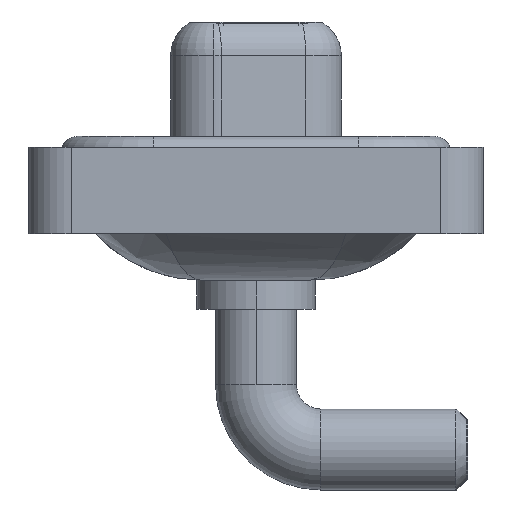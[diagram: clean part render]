
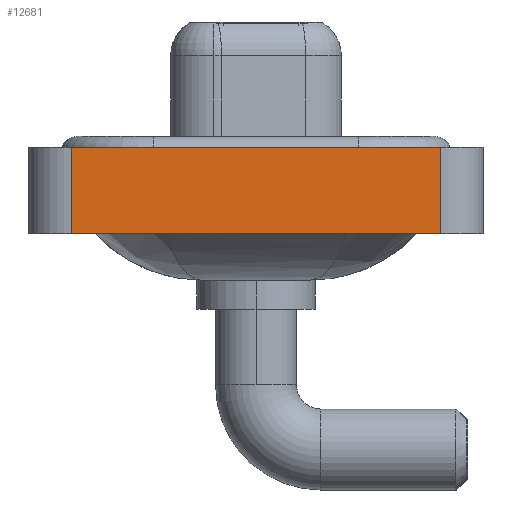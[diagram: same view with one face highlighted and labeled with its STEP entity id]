
A CAD part, left-side view. The second image highlights one B-rep face of the part: STEP entity #12681.
In plain terms, the highlighted planar face has unit normal (-1, 0, 0).
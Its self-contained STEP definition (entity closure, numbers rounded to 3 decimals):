
#26 = ORIENTED_EDGE ( 'NONE', *, *, #15124, .T. ) ;
#262 = VECTOR ( 'NONE', #4863, 1000. ) ;
#936 = PLANE ( 'NONE',  #14161 ) ;
#1154 = ORIENTED_EDGE ( 'NONE', *, *, #9562, .F. ) ;
#1567 = LINE ( 'NONE', #10832, #7258 ) ;
#1940 = VERTEX_POINT ( 'NONE', #12372 ) ;
#2435 = CARTESIAN_POINT ( 'NONE',  ( -7.25, 8.55, -3.6 ) ) ;
#2725 = EDGE_CURVE ( 'NONE', #8722, #10968, #13493, .T. ) ;
#4683 = FACE_OUTER_BOUND ( 'NONE', #9841, .T. ) ;
#4853 = DIRECTION ( 'NONE',  ( -1., 0., 0. ) ) ;
#4863 = DIRECTION ( 'NONE',  ( 0., 0., 1. ) ) ;
#6028 = CARTESIAN_POINT ( 'NONE',  ( -7.25, -8.55, -3.6 ) ) ;
#6979 = CARTESIAN_POINT ( 'NONE',  ( -7.25, 8.55, -3.6 ) ) ;
#7027 = CARTESIAN_POINT ( 'NONE',  ( -7.25, -8.55, -3.6 ) ) ;
#7258 = VECTOR ( 'NONE', #12189, 1000. ) ;
#7540 = DIRECTION ( 'NONE',  ( 0., 0., 1. ) ) ;
#8027 = EDGE_CURVE ( 'NONE', #9073, #1940, #16007, .T. ) ;
#8722 = VERTEX_POINT ( 'NONE', #10783 ) ;
#9073 = VERTEX_POINT ( 'NONE', #2435 ) ;
#9562 = EDGE_CURVE ( 'NONE', #1940, #10968, #16248, .T. ) ;
#9783 = DIRECTION ( 'NONE',  ( 0., -1., 0. ) ) ;
#9841 = EDGE_LOOP ( 'NONE', ( #10234, #1154, #15291, #26 ) ) ;
#10117 = VECTOR ( 'NONE', #7540, 1000. ) ;
#10234 = ORIENTED_EDGE ( 'NONE', *, *, #2725, .T. ) ;
#10783 = CARTESIAN_POINT ( 'NONE',  ( -7.25, -8.55, -3.6 ) ) ;
#10832 = CARTESIAN_POINT ( 'NONE',  ( -7.25, -8.55, -3.6 ) ) ;
#10968 = VERTEX_POINT ( 'NONE', #13185 ) ;
#10972 = CARTESIAN_POINT ( 'NONE',  ( -7.25, -8.55, 0.4 ) ) ;
#12189 = DIRECTION ( 'NONE',  ( 0., -1., 0. ) ) ;
#12372 = CARTESIAN_POINT ( 'NONE',  ( -7.25, 8.55, 0.4 ) ) ;
#12681 = ADVANCED_FACE ( 'NONE', ( #4683 ), #936, .T. ) ;
#13185 = CARTESIAN_POINT ( 'NONE',  ( -7.25, -8.55, 0.4 ) ) ;
#13493 = LINE ( 'NONE', #7027, #10117 ) ;
#14161 = AXIS2_PLACEMENT_3D ( 'NONE', #6028, #4853, #15051 ) ;
#15029 = VECTOR ( 'NONE', #9783, 1000. ) ;
#15051 = DIRECTION ( 'NONE',  ( 0., 0., 1. ) ) ;
#15124 = EDGE_CURVE ( 'NONE', #9073, #8722, #1567, .T. ) ;
#15291 = ORIENTED_EDGE ( 'NONE', *, *, #8027, .F. ) ;
#16007 = LINE ( 'NONE', #6979, #262 ) ;
#16248 = LINE ( 'NONE', #10972, #15029 ) ;
